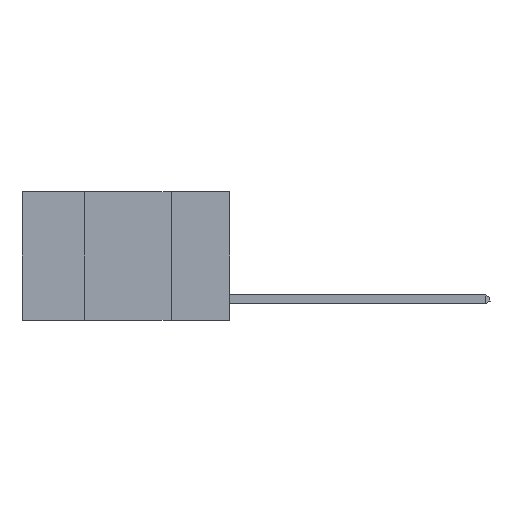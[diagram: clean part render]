
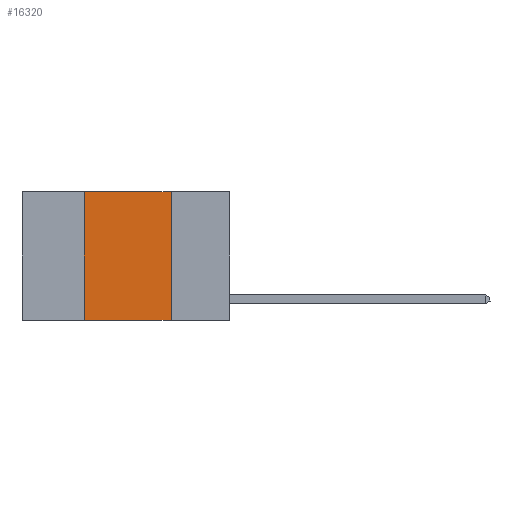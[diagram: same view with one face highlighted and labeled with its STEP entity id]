
A CAD part, left-side view. The second image highlights one B-rep face of the part: STEP entity #16320.
In plain terms, the highlighted planar face has unit normal (-1, 0, 0).
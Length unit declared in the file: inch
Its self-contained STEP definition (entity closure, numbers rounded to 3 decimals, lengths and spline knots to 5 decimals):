
#102 = ORIENTED_EDGE ( 'NONE', *, *, #1096, .T. ) ;
#1096 = EDGE_CURVE ( 'NONE', #3191, #14197, #3980, .T. ) ;
#1688 = VECTOR ( 'NONE', #7096, 39.37008 ) ;
#1801 = LINE ( 'NONE', #9071, #4022 ) ;
#1964 = CARTESIAN_POINT ( 'NONE',  ( 0., 0.6, 0. ) ) ;
#1969 = ORIENTED_EDGE ( 'NONE', *, *, #7230, .F. ) ;
#2881 = CARTESIAN_POINT ( 'NONE',  ( 0., 0.42, 0. ) ) ;
#3191 = VERTEX_POINT ( 'NONE', #4036 ) ;
#3231 = FACE_OUTER_BOUND ( 'NONE', #5753, .T. ) ;
#3449 = AXIS2_PLACEMENT_3D ( 'NONE', #13365, #12097, #15518 ) ;
#3535 = EDGE_CURVE ( 'NONE', #4018, #14197, #11468, .T. ) ;
#3980 = LINE ( 'NONE', #15448, #13194 ) ;
#4018 = VERTEX_POINT ( 'NONE', #6039 ) ;
#4022 = VECTOR ( 'NONE', #10422, 39.37008 ) ;
#4036 = CARTESIAN_POINT ( 'NONE',  ( 0., 0.42, -0.37 ) ) ;
#4567 = ORIENTED_EDGE ( 'NONE', *, *, #7394, .F. ) ;
#5753 = EDGE_LOOP ( 'NONE', ( #13113, #4567, #1969, #102 ) ) ;
#5860 = CARTESIAN_POINT ( 'NONE',  ( 0., 0.17, -0.37 ) ) ;
#6039 = CARTESIAN_POINT ( 'NONE',  ( 0., 0.17, 0. ) ) ;
#7096 = DIRECTION ( 'NONE',  ( 0., -1., 0. ) ) ;
#7230 = EDGE_CURVE ( 'NONE', #3191, #12700, #1801, .T. ) ;
#7394 = EDGE_CURVE ( 'NONE', #12700, #4018, #8563, .T. ) ;
#8279 = PLANE ( 'NONE',  #3449 ) ;
#8563 = LINE ( 'NONE', #1964, #1688 ) ;
#9041 = VECTOR ( 'NONE', #12814, 39.37008 ) ;
#9071 = CARTESIAN_POINT ( 'NONE',  ( 0., 0.42, 0. ) ) ;
#10394 = CARTESIAN_POINT ( 'NONE',  ( 0., 0.17, 0. ) ) ;
#10422 = DIRECTION ( 'NONE',  ( 0., 0., 1. ) ) ;
#11468 = LINE ( 'NONE', #10394, #9041 ) ;
#11855 = DIRECTION ( 'NONE',  ( 0., -1., 0. ) ) ;
#12097 = DIRECTION ( 'NONE',  ( 1., 0., 0. ) ) ;
#12700 = VERTEX_POINT ( 'NONE', #2881 ) ;
#12814 = DIRECTION ( 'NONE',  ( 0., 0., -1. ) ) ;
#13113 = ORIENTED_EDGE ( 'NONE', *, *, #3535, .F. ) ;
#13194 = VECTOR ( 'NONE', #11855, 39.37008 ) ;
#13365 = CARTESIAN_POINT ( 'NONE',  ( 0., 0.6, 0. ) ) ;
#14197 = VERTEX_POINT ( 'NONE', #5860 ) ;
#15448 = CARTESIAN_POINT ( 'NONE',  ( 0., 0.6, -0.37 ) ) ;
#15518 = DIRECTION ( 'NONE',  ( 0., 0., -1. ) ) ;
#16320 = ADVANCED_FACE ( 'NONE', ( #3231 ), #8279, .F. ) ;
